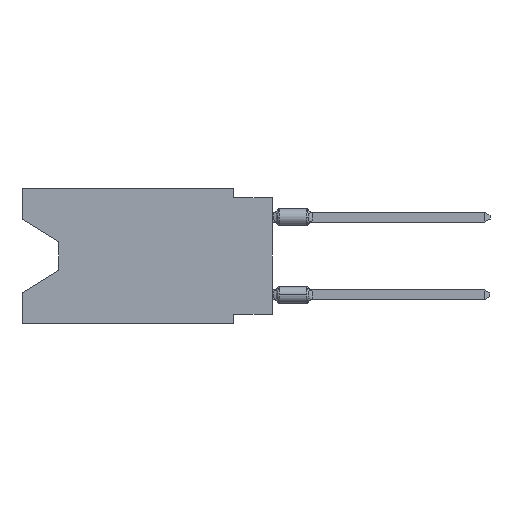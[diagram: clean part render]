
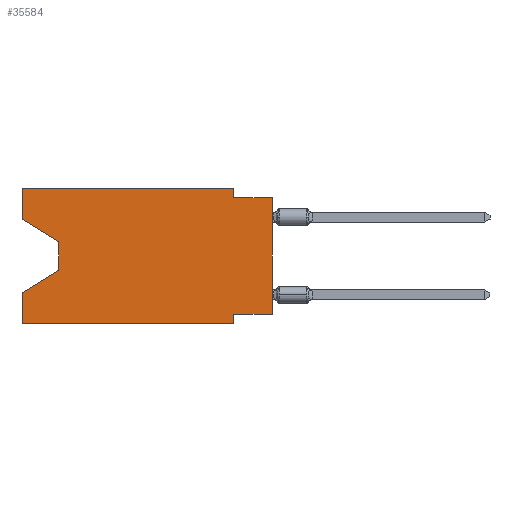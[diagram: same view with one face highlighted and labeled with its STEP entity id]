
A CAD part, left-side view. The second image highlights one B-rep face of the part: STEP entity #35584.
In plain terms, the highlighted planar face has unit normal (-1, 0, 0).
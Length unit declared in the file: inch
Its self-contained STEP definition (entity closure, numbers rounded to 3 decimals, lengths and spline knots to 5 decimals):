
#248 = EDGE_CURVE ( 'NONE', #43473, #15079, #34403, .T. ) ;
#351 = VECTOR ( 'NONE', #42196, 39.37008 ) ;
#620 = LINE ( 'NONE', #46646, #43456 ) ;
#903 = CARTESIAN_POINT ( 'NONE',  ( 0., 0.645, -0.26975 ) ) ;
#1216 = CARTESIAN_POINT ( 'NONE',  ( 0., 0.1, -0.35 ) ) ;
#1900 = CARTESIAN_POINT ( 'NONE',  ( 0., 0.55, -0.138 ) ) ;
#2526 = LINE ( 'NONE', #18198, #18409 ) ;
#2759 = EDGE_CURVE ( 'NONE', #49603, #25255, #620, .T. ) ;
#3146 = ORIENTED_EDGE ( 'NONE', *, *, #33909, .F. ) ;
#3430 = EDGE_LOOP ( 'NONE', ( #18072, #22621, #9610, #3996, #9418, #3146, #11852, #42038, #7136, #24287, #27109, #20385 ) ) ;
#3743 = LINE ( 'NONE', #34866, #351 ) ;
#3797 = VERTEX_POINT ( 'NONE', #23421 ) ;
#3996 = ORIENTED_EDGE ( 'NONE', *, *, #21102, .F. ) ;
#4030 = CARTESIAN_POINT ( 'NONE',  ( 0., 0.55, -0.212 ) ) ;
#4287 = EDGE_CURVE ( 'NONE', #13579, #49603, #2526, .T. ) ;
#4811 = EDGE_CURVE ( 'NONE', #9212, #25255, #19718, .T. ) ;
#5308 = CARTESIAN_POINT ( 'NONE',  ( 0., 0., -0.325 ) ) ;
#5743 = DIRECTION ( 'NONE',  ( 0., -1., 0. ) ) ;
#5759 = VECTOR ( 'NONE', #39616, 39.37008 ) ;
#5973 = CARTESIAN_POINT ( 'NONE',  ( 0., 0.645, 0. ) ) ;
#5982 = DIRECTION ( 'NONE',  ( 0., 0., -1. ) ) ;
#6318 = CARTESIAN_POINT ( 'NONE',  ( 0., 0.645, -0.08025 ) ) ;
#6533 = EDGE_CURVE ( 'NONE', #37332, #22074, #3743, .T. ) ;
#7136 = ORIENTED_EDGE ( 'NONE', *, *, #2759, .F. ) ;
#7870 = DIRECTION ( 'NONE',  ( 0., -1., 0. ) ) ;
#8233 = CARTESIAN_POINT ( 'NONE',  ( 0., 0., -0.325 ) ) ;
#9212 = VERTEX_POINT ( 'NONE', #5308 ) ;
#9418 = ORIENTED_EDGE ( 'NONE', *, *, #6533, .T. ) ;
#9610 = ORIENTED_EDGE ( 'NONE', *, *, #46531, .T. ) ;
#9781 = LINE ( 'NONE', #48458, #19203 ) ;
#11852 = ORIENTED_EDGE ( 'NONE', *, *, #37515, .F. ) ;
#12806 = PLANE ( 'NONE',  #25763 ) ;
#13579 = VERTEX_POINT ( 'NONE', #49736 ) ;
#13946 = DIRECTION ( 'NONE',  ( 0., 0.855, -0.519 ) ) ;
#14199 = VECTOR ( 'NONE', #18220, 39.37008 ) ;
#14751 = LINE ( 'NONE', #31196, #40058 ) ;
#15079 = VERTEX_POINT ( 'NONE', #4030 ) ;
#16110 = CARTESIAN_POINT ( 'NONE',  ( 0., 0.645, 0. ) ) ;
#16315 = LINE ( 'NONE', #8233, #5759 ) ;
#16577 = LINE ( 'NONE', #16832, #46054 ) ;
#16832 = CARTESIAN_POINT ( 'NONE',  ( 0., 0.645, 0. ) ) ;
#17747 = CARTESIAN_POINT ( 'NONE',  ( 0., 0.55, -0.212 ) ) ;
#18072 = ORIENTED_EDGE ( 'NONE', *, *, #41812, .T. ) ;
#18198 = CARTESIAN_POINT ( 'NONE',  ( 0., 0.1, 0. ) ) ;
#18220 = DIRECTION ( 'NONE',  ( 0., 0., -1. ) ) ;
#18409 = VECTOR ( 'NONE', #37432, 39.37008 ) ;
#19203 = VECTOR ( 'NONE', #5982, 39.37008 ) ;
#19718 = LINE ( 'NONE', #27309, #39613 ) ;
#20385 = ORIENTED_EDGE ( 'NONE', *, *, #30121, .F. ) ;
#20661 = LINE ( 'NONE', #5973, #46712 ) ;
#21102 = EDGE_CURVE ( 'NONE', #37332, #44291, #14751, .T. ) ;
#22074 = VERTEX_POINT ( 'NONE', #1216 ) ;
#22621 = ORIENTED_EDGE ( 'NONE', *, *, #248, .T. ) ;
#23421 = CARTESIAN_POINT ( 'NONE',  ( 0., 0.1, -0.325 ) ) ;
#23448 = CARTESIAN_POINT ( 'NONE',  ( 0., 0.645, -0.08025 ) ) ;
#24287 = ORIENTED_EDGE ( 'NONE', *, *, #4287, .F. ) ;
#25255 = VERTEX_POINT ( 'NONE', #31624 ) ;
#25457 = VERTEX_POINT ( 'NONE', #6318 ) ;
#25763 = AXIS2_PLACEMENT_3D ( 'NONE', #16110, #42931, #46950 ) ;
#26860 = CARTESIAN_POINT ( 'NONE',  ( 0., 0.645, 0. ) ) ;
#27109 = ORIENTED_EDGE ( 'NONE', *, *, #32657, .F. ) ;
#27309 = CARTESIAN_POINT ( 'NONE',  ( 0., 0., 0. ) ) ;
#30121 = EDGE_CURVE ( 'NONE', #25457, #39137, #16577, .T. ) ;
#30847 = CARTESIAN_POINT ( 'NONE',  ( 0., 0.55, -0.138 ) ) ;
#31196 = CARTESIAN_POINT ( 'NONE',  ( 0., 0.645, 0. ) ) ;
#31624 = CARTESIAN_POINT ( 'NONE',  ( 0., 0., -0.025 ) ) ;
#32657 = EDGE_CURVE ( 'NONE', #39137, #13579, #20661, .T. ) ;
#33909 = EDGE_CURVE ( 'NONE', #3797, #22074, #9781, .T. ) ;
#34195 = VECTOR ( 'NONE', #39900, 39.37008 ) ;
#34403 = LINE ( 'NONE', #30847, #14199 ) ;
#34662 = DIRECTION ( 'NONE',  ( 0., 0., 1. ) ) ;
#34866 = CARTESIAN_POINT ( 'NONE',  ( 0., 0.645, -0.35 ) ) ;
#35353 = LINE ( 'NONE', #23448, #34195 ) ;
#35584 = ADVANCED_FACE ( 'NONE', ( #41985 ), #12806, .F. ) ;
#37332 = VERTEX_POINT ( 'NONE', #45416 ) ;
#37432 = DIRECTION ( 'NONE',  ( 0., 0., -1. ) ) ;
#37515 = EDGE_CURVE ( 'NONE', #9212, #3797, #16315, .T. ) ;
#37978 = LINE ( 'NONE', #17747, #40866 ) ;
#39137 = VERTEX_POINT ( 'NONE', #26860 ) ;
#39613 = VECTOR ( 'NONE', #34662, 39.37008 ) ;
#39616 = DIRECTION ( 'NONE',  ( 0., 1., 0. ) ) ;
#39617 = DIRECTION ( 'NONE',  ( 0., 0., 1. ) ) ;
#39900 = DIRECTION ( 'NONE',  ( 0., -0.855, -0.519 ) ) ;
#40058 = VECTOR ( 'NONE', #42080, 39.37008 ) ;
#40866 = VECTOR ( 'NONE', #13946, 39.37008 ) ;
#41812 = EDGE_CURVE ( 'NONE', #25457, #43473, #35353, .T. ) ;
#41985 = FACE_OUTER_BOUND ( 'NONE', #3430, .T. ) ;
#42038 = ORIENTED_EDGE ( 'NONE', *, *, #4811, .T. ) ;
#42080 = DIRECTION ( 'NONE',  ( 0., 0., 1. ) ) ;
#42196 = DIRECTION ( 'NONE',  ( 0., -1., 0. ) ) ;
#42931 = DIRECTION ( 'NONE',  ( 1., 0., 0. ) ) ;
#43456 = VECTOR ( 'NONE', #7870, 39.37008 ) ;
#43473 = VERTEX_POINT ( 'NONE', #1900 ) ;
#44291 = VERTEX_POINT ( 'NONE', #903 ) ;
#45416 = CARTESIAN_POINT ( 'NONE',  ( 0., 0.645, -0.35 ) ) ;
#46054 = VECTOR ( 'NONE', #39617, 39.37008 ) ;
#46531 = EDGE_CURVE ( 'NONE', #15079, #44291, #37978, .T. ) ;
#46646 = CARTESIAN_POINT ( 'NONE',  ( 0., 0., -0.025 ) ) ;
#46712 = VECTOR ( 'NONE', #5743, 39.37008 ) ;
#46950 = DIRECTION ( 'NONE',  ( 0., 0., -1. ) ) ;
#48458 = CARTESIAN_POINT ( 'NONE',  ( 0., 0.1, -0.35 ) ) ;
#48805 = CARTESIAN_POINT ( 'NONE',  ( 0., 0.1, -0.025 ) ) ;
#49603 = VERTEX_POINT ( 'NONE', #48805 ) ;
#49736 = CARTESIAN_POINT ( 'NONE',  ( 0., 0.1, 0. ) ) ;
